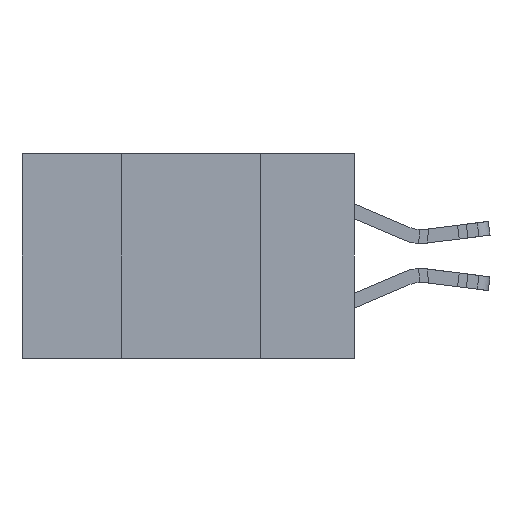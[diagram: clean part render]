
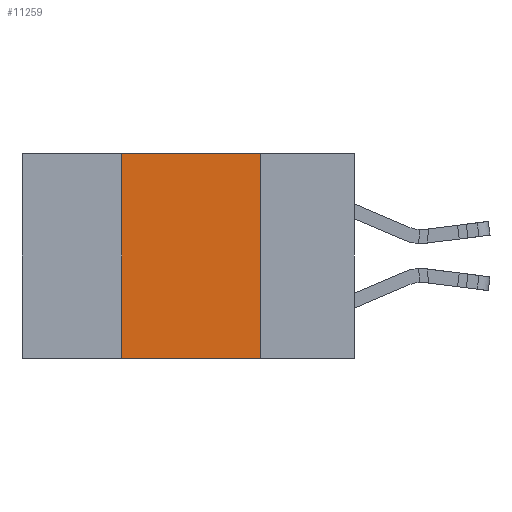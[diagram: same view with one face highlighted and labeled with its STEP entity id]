
A CAD part, left-side view. The second image highlights one B-rep face of the part: STEP entity #11259.
In plain terms, the highlighted planar face has unit normal (-1, 0, 0).
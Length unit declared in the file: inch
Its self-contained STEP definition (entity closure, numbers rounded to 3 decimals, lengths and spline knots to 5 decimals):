
#490 = CARTESIAN_POINT ( 'NONE',  ( 0., 0.6, -0.37 ) ) ;
#927 = VERTEX_POINT ( 'NONE', #18308 ) ;
#955 = VECTOR ( 'NONE', #2084, 39.37008 ) ;
#2084 = DIRECTION ( 'NONE',  ( 0., 0., 1. ) ) ;
#2264 = VERTEX_POINT ( 'NONE', #6954 ) ;
#2296 = CARTESIAN_POINT ( 'NONE',  ( 0., 0.6, 0. ) ) ;
#2600 = CARTESIAN_POINT ( 'NONE',  ( 0., 0.17, 0. ) ) ;
#3274 = DIRECTION ( 'NONE',  ( 1., 0., 0. ) ) ;
#3762 = CARTESIAN_POINT ( 'NONE',  ( 0., 0.6, 0. ) ) ;
#4707 = CARTESIAN_POINT ( 'NONE',  ( 0., 0.17, -0.37 ) ) ;
#4785 = AXIS2_PLACEMENT_3D ( 'NONE', #3762, #3274, #11058 ) ;
#5182 = LINE ( 'NONE', #4707, #14540 ) ;
#5371 = FACE_OUTER_BOUND ( 'NONE', #22497, .T. ) ;
#5743 = VERTEX_POINT ( 'NONE', #19578 ) ;
#6314 = EDGE_CURVE ( 'NONE', #14513, #5743, #5182, .T. ) ;
#6811 = VECTOR ( 'NONE', #22388, 39.37008 ) ;
#6954 = CARTESIAN_POINT ( 'NONE',  ( 0., 0.42, 0. ) ) ;
#7469 = PLANE ( 'NONE',  #4785 ) ;
#9772 = DIRECTION ( 'NONE',  ( 0., -1., 0. ) ) ;
#11058 = DIRECTION ( 'NONE',  ( 0., 0., -1. ) ) ;
#11120 = VECTOR ( 'NONE', #9772, 39.37008 ) ;
#11259 = ADVANCED_FACE ( 'NONE', ( #5371 ), #7469, .F. ) ;
#11344 = ORIENTED_EDGE ( 'NONE', *, *, #11759, .T. ) ;
#11759 = EDGE_CURVE ( 'NONE', #927, #5743, #23008, .T. ) ;
#12818 = ORIENTED_EDGE ( 'NONE', *, *, #14818, .F. ) ;
#14513 = VERTEX_POINT ( 'NONE', #2600 ) ;
#14540 = VECTOR ( 'NONE', #14575, 39.37008 ) ;
#14575 = DIRECTION ( 'NONE',  ( 0., 0., -1. ) ) ;
#14818 = EDGE_CURVE ( 'NONE', #927, #2264, #20754, .T. ) ;
#18308 = CARTESIAN_POINT ( 'NONE',  ( 0., 0.42, -0.37 ) ) ;
#18432 = LINE ( 'NONE', #2296, #6811 ) ;
#19437 = ORIENTED_EDGE ( 'NONE', *, *, #6314, .F. ) ;
#19578 = CARTESIAN_POINT ( 'NONE',  ( 0., 0.17, -0.37 ) ) ;
#20041 = EDGE_CURVE ( 'NONE', #2264, #14513, #18432, .T. ) ;
#20628 = CARTESIAN_POINT ( 'NONE',  ( 0., 0.42, -0.37 ) ) ;
#20754 = LINE ( 'NONE', #20628, #955 ) ;
#22388 = DIRECTION ( 'NONE',  ( 0., -1., 0. ) ) ;
#22497 = EDGE_LOOP ( 'NONE', ( #19437, #22849, #12818, #11344 ) ) ;
#22849 = ORIENTED_EDGE ( 'NONE', *, *, #20041, .F. ) ;
#23008 = LINE ( 'NONE', #490, #11120 ) ;
